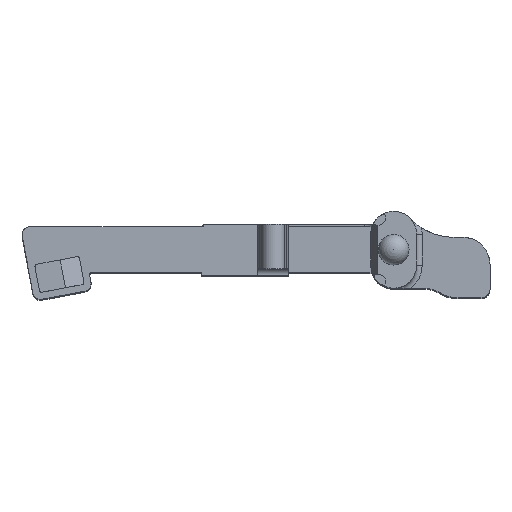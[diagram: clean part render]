
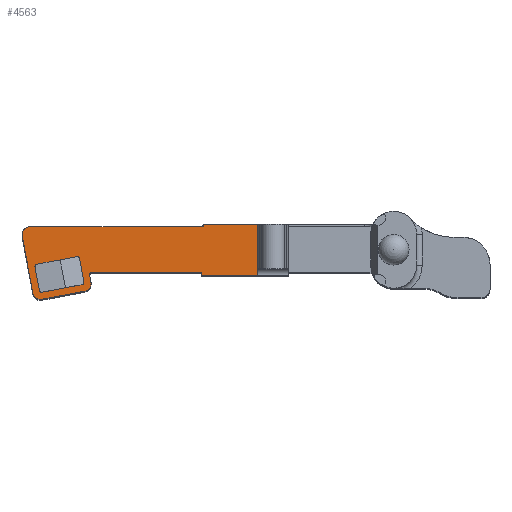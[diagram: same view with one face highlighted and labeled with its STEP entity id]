
A CAD part, top view. The second image highlights one B-rep face of the part: STEP entity #4563.
In plain terms, the highlighted planar face has unit normal (0, 0, 1).
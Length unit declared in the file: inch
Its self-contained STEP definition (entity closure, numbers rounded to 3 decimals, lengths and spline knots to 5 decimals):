
#25=FACE_BOUND('',#1469,.T.);
#118=PLANE('',#4867);
#287=LINE('',#6993,#705);
#288=LINE('',#6995,#706);
#289=LINE('',#6997,#707);
#290=LINE('',#6999,#708);
#291=LINE('',#7003,#709);
#292=LINE('',#7007,#710);
#293=LINE('',#7011,#711);
#294=LINE('',#7015,#712);
#295=LINE('',#7017,#713);
#296=LINE('',#7018,#714);
#297=LINE('',#7023,#715);
#298=LINE('',#7027,#716);
#299=LINE('',#7031,#717);
#300=LINE('',#7034,#718);
#705=VECTOR('',#5487,0.3937);
#706=VECTOR('',#5488,0.3937);
#707=VECTOR('',#5489,0.3937);
#708=VECTOR('',#5490,0.3937);
#709=VECTOR('',#5493,0.3937);
#710=VECTOR('',#5496,0.3937);
#711=VECTOR('',#5499,0.3937);
#712=VECTOR('',#5502,0.3937);
#713=VECTOR('',#5503,0.3937);
#714=VECTOR('',#5504,0.3937);
#715=VECTOR('',#5507,0.3937);
#716=VECTOR('',#5510,0.3937);
#717=VECTOR('',#5513,0.3937);
#718=VECTOR('',#5516,0.3937);
#1216=FACE_OUTER_BOUND('',#1468,.T.);
#1468=EDGE_LOOP('',(#3271,#3272,#3273,#3274,#3275,#3276,#3277,#3278,#3279,
#3280,#3281,#3282,#3283,#3284));
#1469=EDGE_LOOP('',(#3285,#3286,#3287,#3288,#3289,#3290,#3291,#3292));
#1763=CIRCLE('',#4868,0.05);
#1764=CIRCLE('',#4869,0.05);
#1765=CIRCLE('',#4870,0.05);
#1766=CIRCLE('',#4871,0.01);
#1767=CIRCLE('',#4872,0.015);
#1768=CIRCLE('',#4873,0.015);
#1769=CIRCLE('',#4874,0.015);
#1770=CIRCLE('',#4875,0.015);
#1991=VERTEX_POINT('',#6988);
#1992=VERTEX_POINT('',#6992);
#1993=VERTEX_POINT('',#6994);
#1994=VERTEX_POINT('',#6996);
#1995=VERTEX_POINT('',#6998);
#1996=VERTEX_POINT('',#7000);
#1997=VERTEX_POINT('',#7002);
#1998=VERTEX_POINT('',#7004);
#1999=VERTEX_POINT('',#7006);
#2000=VERTEX_POINT('',#7008);
#2001=VERTEX_POINT('',#7010);
#2002=VERTEX_POINT('',#7012);
#2003=VERTEX_POINT('',#7014);
#2004=VERTEX_POINT('',#7016);
#2005=VERTEX_POINT('',#7019);
#2006=VERTEX_POINT('',#7020);
#2007=VERTEX_POINT('',#7022);
#2008=VERTEX_POINT('',#7024);
#2009=VERTEX_POINT('',#7026);
#2010=VERTEX_POINT('',#7028);
#2011=VERTEX_POINT('',#7030);
#2012=VERTEX_POINT('',#7032);
#2492=EDGE_CURVE('',#1991,#1992,#287,.T.);
#2493=EDGE_CURVE('',#1993,#1992,#288,.T.);
#2494=EDGE_CURVE('',#1994,#1993,#289,.T.);
#2495=EDGE_CURVE('',#1995,#1994,#290,.T.);
#2496=EDGE_CURVE('',#1996,#1995,#1763,.T.);
#2497=EDGE_CURVE('',#1997,#1996,#291,.T.);
#2498=EDGE_CURVE('',#1998,#1997,#1764,.T.);
#2499=EDGE_CURVE('',#1999,#1998,#292,.T.);
#2500=EDGE_CURVE('',#2000,#1999,#1765,.T.);
#2501=EDGE_CURVE('',#2001,#2000,#293,.T.);
#2502=EDGE_CURVE('',#2002,#2001,#1766,.T.);
#2503=EDGE_CURVE('',#2003,#2002,#294,.T.);
#2504=EDGE_CURVE('',#2004,#2003,#295,.T.);
#2505=EDGE_CURVE('',#1991,#2004,#296,.T.);
#2506=EDGE_CURVE('',#2005,#2006,#1767,.T.);
#2507=EDGE_CURVE('',#2006,#2007,#297,.T.);
#2508=EDGE_CURVE('',#2007,#2008,#1768,.T.);
#2509=EDGE_CURVE('',#2008,#2009,#298,.T.);
#2510=EDGE_CURVE('',#2009,#2010,#1769,.T.);
#2511=EDGE_CURVE('',#2010,#2011,#299,.T.);
#2512=EDGE_CURVE('',#2011,#2012,#1770,.T.);
#2513=EDGE_CURVE('',#2012,#2005,#300,.T.);
#3271=ORIENTED_EDGE('',*,*,#2492,.T.);
#3272=ORIENTED_EDGE('',*,*,#2493,.F.);
#3273=ORIENTED_EDGE('',*,*,#2494,.F.);
#3274=ORIENTED_EDGE('',*,*,#2495,.F.);
#3275=ORIENTED_EDGE('',*,*,#2496,.F.);
#3276=ORIENTED_EDGE('',*,*,#2497,.F.);
#3277=ORIENTED_EDGE('',*,*,#2498,.F.);
#3278=ORIENTED_EDGE('',*,*,#2499,.F.);
#3279=ORIENTED_EDGE('',*,*,#2500,.F.);
#3280=ORIENTED_EDGE('',*,*,#2501,.F.);
#3281=ORIENTED_EDGE('',*,*,#2502,.F.);
#3282=ORIENTED_EDGE('',*,*,#2503,.F.);
#3283=ORIENTED_EDGE('',*,*,#2504,.F.);
#3284=ORIENTED_EDGE('',*,*,#2505,.F.);
#3285=ORIENTED_EDGE('',*,*,#2506,.T.);
#3286=ORIENTED_EDGE('',*,*,#2507,.T.);
#3287=ORIENTED_EDGE('',*,*,#2508,.T.);
#3288=ORIENTED_EDGE('',*,*,#2509,.T.);
#3289=ORIENTED_EDGE('',*,*,#2510,.T.);
#3290=ORIENTED_EDGE('',*,*,#2511,.T.);
#3291=ORIENTED_EDGE('',*,*,#2512,.T.);
#3292=ORIENTED_EDGE('',*,*,#2513,.T.);
#4563=ADVANCED_FACE('',(#1216,#25),#118,.F.);
#4867=AXIS2_PLACEMENT_3D('',#6991,#5485,#5486);
#4868=AXIS2_PLACEMENT_3D('',#7001,#5491,#5492);
#4869=AXIS2_PLACEMENT_3D('',#7005,#5494,#5495);
#4870=AXIS2_PLACEMENT_3D('',#7009,#5497,#5498);
#4871=AXIS2_PLACEMENT_3D('',#7013,#5500,#5501);
#4872=AXIS2_PLACEMENT_3D('',#7021,#5505,#5506);
#4873=AXIS2_PLACEMENT_3D('',#7025,#5508,#5509);
#4874=AXIS2_PLACEMENT_3D('',#7029,#5511,#5512);
#4875=AXIS2_PLACEMENT_3D('',#7033,#5514,#5515);
#5485=DIRECTION('center_axis',(0.,0.,
-1.));
#5486=DIRECTION('ref_axis',(-1.,0.,0.));
#5487=DIRECTION('',(0.,1.,0.));
#5488=DIRECTION('',(1.,0.,0.));
#5489=DIRECTION('',(0.,1.,0.));
#5490=DIRECTION('',(1.,0.,0.));
#5491=DIRECTION('center_axis',(0.,0.,
-1.));
#5492=DIRECTION('ref_axis',(-0.983,-0.185,0.));
#5493=DIRECTION('',(-0.185,0.983,0.));
#5494=DIRECTION('center_axis',(0.,0.,
-1.));
#5495=DIRECTION('ref_axis',(0.185,-0.983,0.));
#5496=DIRECTION('',(-0.983,-0.185,0.));
#5497=DIRECTION('center_axis',(0.,0.,
-1.));
#5498=DIRECTION('ref_axis',(0.983,0.185,0.));
#5499=DIRECTION('',(0.185,-0.983,0.));
#5500=DIRECTION('center_axis',(0.,0.,
1.));
#5501=DIRECTION('ref_axis',(0.983,0.185,0.));
#5502=DIRECTION('',(-1.,0.,0.));
#5503=DIRECTION('',(0.,1.,0.));
#5504=DIRECTION('',(-1.,0.,0.));
#5505=DIRECTION('center_axis',(0.,0.,
-1.));
#5506=DIRECTION('ref_axis',(0.185,-0.983,0.));
#5507=DIRECTION('',(0.185,-0.983,0.));
#5508=DIRECTION('center_axis',(0.,0.,
-1.));
#5509=DIRECTION('ref_axis',(-0.983,-0.185,0.));
#5510=DIRECTION('',(-0.983,-0.185,0.));
#5511=DIRECTION('center_axis',(0.,0.,
-1.));
#5512=DIRECTION('ref_axis',(-0.185,0.983,0.));
#5513=DIRECTION('',(-0.185,0.983,0.));
#5514=DIRECTION('center_axis',(0.,0.,
-1.));
#5515=DIRECTION('ref_axis',(0.983,0.185,0.));
#5516=DIRECTION('',(0.983,0.185,0.));
#6988=CARTESIAN_POINT('',(2.20472,-0.71993,-3.96678));
#6991=CARTESIAN_POINT('Origin',(1.92698,-0.57141,-3.96678));
#6992=CARTESIAN_POINT('',(2.20472,-0.38993,-3.96678));
#6993=CARTESIAN_POINT('',(2.20472,-0.48067,-3.96678));
#6994=CARTESIAN_POINT('',(1.84964,-0.38993,-3.96678));
#6995=CARTESIAN_POINT('',(1.84964,-0.38993,-3.96678));
#6996=CARTESIAN_POINT('',(1.84964,-0.40493,-3.96678));
#6997=CARTESIAN_POINT('',(1.84964,-0.40493,-3.96678));
#6998=CARTESIAN_POINT('',(0.71686,-0.40493,-3.96678));
#6999=CARTESIAN_POINT('',(0.71686,-0.40493,-3.96678));
#7000=CARTESIAN_POINT('',(0.66772,-0.46417,-3.96678));
#7001=CARTESIAN_POINT('Origin',(0.71686,-0.45493,-3.96678));
#7002=CARTESIAN_POINT('',(0.7379,-0.83735,-3.96678));
#7003=CARTESIAN_POINT('',(0.7379,-0.83735,-3.96678));
#7004=CARTESIAN_POINT('',(0.79628,-0.87725,-3.96678));
#7005=CARTESIAN_POINT('Origin',(0.78704,-0.82811,-3.96678));
#7006=CARTESIAN_POINT('',(1.07637,-0.82458,-3.96678));
#7007=CARTESIAN_POINT('',(1.07637,-0.82458,-3.96678));
#7008=CARTESIAN_POINT('',(1.11626,-0.7662,-3.96678));
#7009=CARTESIAN_POINT('Origin',(1.06713,-0.77544,-3.96678));
#7010=CARTESIAN_POINT('',(1.10697,-0.71678,-3.96678));
#7011=CARTESIAN_POINT('',(1.10697,-0.71678,-3.96678));
#7012=CARTESIAN_POINT('',(1.1168,-0.70493,-3.96678));
#7013=CARTESIAN_POINT('Origin',(1.1168,-0.71493,-3.96678));
#7014=CARTESIAN_POINT('',(1.83964,-0.70493,-3.96678));
#7015=CARTESIAN_POINT('',(1.83964,-0.70493,-3.96678));
#7016=CARTESIAN_POINT('',(1.83964,-0.71993,-3.96678));
#7017=CARTESIAN_POINT('',(1.83964,-0.71993,-3.96678));
#7018=CARTESIAN_POINT('',(2.29964,-0.71993,-3.96678));
#7019=CARTESIAN_POINT('',(1.02403,-0.60039,-3.96678));
#7020=CARTESIAN_POINT('',(1.04155,-0.61236,-3.96678));
#7021=CARTESIAN_POINT('Origin',(1.0268,-0.61513,-3.96678));
#7022=CARTESIAN_POINT('',(1.07019,-0.76469,-3.96678));
#7023=CARTESIAN_POINT('',(1.06727,-0.74916,-3.96678));
#7024=CARTESIAN_POINT('',(1.05822,-0.7822,-3.96678));
#7025=CARTESIAN_POINT('Origin',(1.05545,-0.76746,-3.96678));
#7026=CARTESIAN_POINT('',(0.79779,-0.83118,-3.96678));
#7027=CARTESIAN_POINT('',(1.36669,-0.72419,-3.96678));
#7028=CARTESIAN_POINT('',(0.78027,-0.81921,-3.96678));
#7029=CARTESIAN_POINT('Origin',(0.79502,-0.81643,-3.96678));
#7030=CARTESIAN_POINT('',(0.75163,-0.66688,-3.96678));
#7031=CARTESIAN_POINT('',(0.76303,-0.72751,-3.96678));
#7032=CARTESIAN_POINT('',(0.7636,-0.64936,-3.96678));
#7033=CARTESIAN_POINT('Origin',(0.76637,-0.6641,-3.96678));
#7034=CARTESIAN_POINT('',(1.46272,-0.51789,-3.96678));
